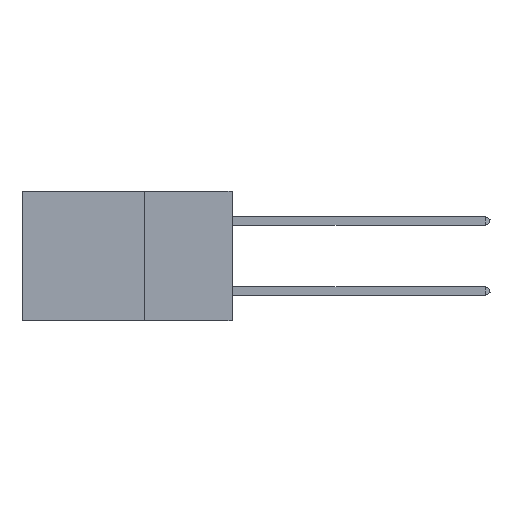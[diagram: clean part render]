
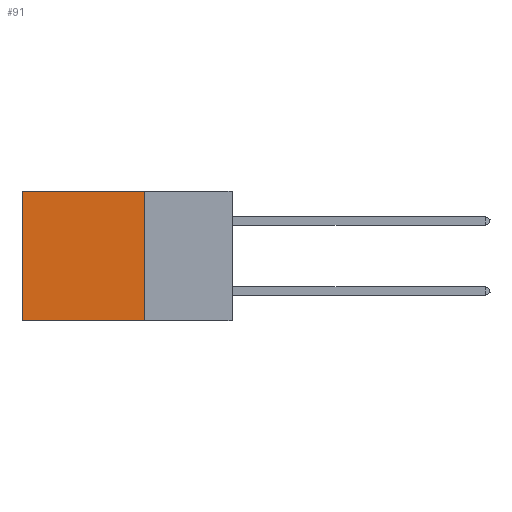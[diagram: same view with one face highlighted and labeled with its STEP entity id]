
A CAD part, left-side view. The second image highlights one B-rep face of the part: STEP entity #91.
In plain terms, the highlighted planar face has unit normal (-1, 0, 0).
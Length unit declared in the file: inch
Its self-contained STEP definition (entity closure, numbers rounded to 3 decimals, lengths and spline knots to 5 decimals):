
#91 = ADVANCED_FACE ( 'NONE', ( #3426 ), #20625, .F. ) ;
#860 = ORIENTED_EDGE ( 'NONE', *, *, #17073, .T. ) ;
#1846 = ORIENTED_EDGE ( 'NONE', *, *, #10477, .F. ) ;
#2188 = VECTOR ( 'NONE', #18855, 39.37008 ) ;
#3426 = FACE_OUTER_BOUND ( 'NONE', #7065, .T. ) ;
#5383 = VERTEX_POINT ( 'NONE', #11616 ) ;
#6131 = ORIENTED_EDGE ( 'NONE', *, *, #17898, .T. ) ;
#6670 = DIRECTION ( 'NONE',  ( 0., 0., -1. ) ) ;
#6779 = DIRECTION ( 'NONE',  ( 0., 1., 0. ) ) ;
#7065 = EDGE_LOOP ( 'NONE', ( #860, #16507, #1846, #6131 ) ) ;
#7844 = VECTOR ( 'NONE', #6779, 39.37008 ) ;
#8381 = CARTESIAN_POINT ( 'NONE',  ( 0.2875, 0.25, 0. ) ) ;
#9872 = LINE ( 'NONE', #13903, #7844 ) ;
#10332 = DIRECTION ( 'NONE',  ( 1., 0., 0. ) ) ;
#10477 = EDGE_CURVE ( 'NONE', #12440, #18132, #18404, .T. ) ;
#10819 = CARTESIAN_POINT ( 'NONE',  ( 0.2875, 0.6, 0. ) ) ;
#10873 = DIRECTION ( 'NONE',  ( 0., 0., -1. ) ) ;
#10947 = AXIS2_PLACEMENT_3D ( 'NONE', #8381, #10332, #13806 ) ;
#10959 = VECTOR ( 'NONE', #10873, 39.37008 ) ;
#11616 = CARTESIAN_POINT ( 'NONE',  ( 0.2875, 0.6, -0.37 ) ) ;
#11967 = EDGE_CURVE ( 'NONE', #18132, #5383, #15259, .T. ) ;
#12440 = VERTEX_POINT ( 'NONE', #19407 ) ;
#12480 = LINE ( 'NONE', #14335, #13352 ) ;
#13352 = VECTOR ( 'NONE', #6670, 39.37008 ) ;
#13806 = DIRECTION ( 'NONE',  ( 0., 0., -1. ) ) ;
#13903 = CARTESIAN_POINT ( 'NONE',  ( 0.2875, 0.25, 0. ) ) ;
#14335 = CARTESIAN_POINT ( 'NONE',  ( 0.2875, 0.6, 0. ) ) ;
#15259 = LINE ( 'NONE', #17119, #2188 ) ;
#16313 = CARTESIAN_POINT ( 'NONE',  ( 0.2875, 0.25, 0. ) ) ;
#16507 = ORIENTED_EDGE ( 'NONE', *, *, #11967, .F. ) ;
#16848 = VERTEX_POINT ( 'NONE', #10819 ) ;
#17073 = EDGE_CURVE ( 'NONE', #16848, #5383, #12480, .T. ) ;
#17119 = CARTESIAN_POINT ( 'NONE',  ( 0.2875, 0.25, -0.37 ) ) ;
#17898 = EDGE_CURVE ( 'NONE', #12440, #16848, #9872, .T. ) ;
#18132 = VERTEX_POINT ( 'NONE', #21842 ) ;
#18404 = LINE ( 'NONE', #16313, #10959 ) ;
#18855 = DIRECTION ( 'NONE',  ( 0., 1., 0. ) ) ;
#19407 = CARTESIAN_POINT ( 'NONE',  ( 0.2875, 0.25, 0. ) ) ;
#20625 = PLANE ( 'NONE',  #10947 ) ;
#21842 = CARTESIAN_POINT ( 'NONE',  ( 0.2875, 0.25, -0.37 ) ) ;
